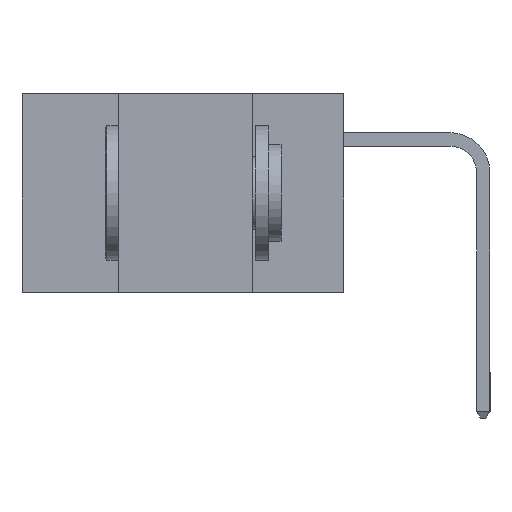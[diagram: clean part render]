
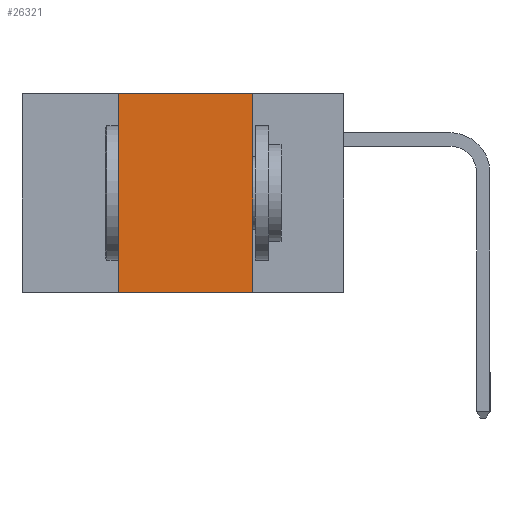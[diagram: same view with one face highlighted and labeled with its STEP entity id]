
A CAD part, left-side view. The second image highlights one B-rep face of the part: STEP entity #26321.
In plain terms, the highlighted planar face has unit normal (-1, 0, 0).
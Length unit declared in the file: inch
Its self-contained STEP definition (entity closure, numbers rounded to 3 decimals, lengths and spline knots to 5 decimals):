
#24 = LINE ( 'NONE', #15750, #25617 ) ;
#314 = FACE_OUTER_BOUND ( 'NONE', #26696, .T. ) ;
#1170 = EDGE_CURVE ( 'NONE', #27812, #8959, #24, .T. ) ;
#1636 = ORIENTED_EDGE ( 'NONE', *, *, #12456, .F. ) ;
#3092 = EDGE_CURVE ( 'NONE', #28679, #8959, #13133, .T. ) ;
#3918 = ORIENTED_EDGE ( 'NONE', *, *, #3092, .T. ) ;
#4288 = DIRECTION ( 'NONE',  ( 0., 0., -1. ) ) ;
#5639 = VECTOR ( 'NONE', #26597, 39.37008 ) ;
#6387 = LINE ( 'NONE', #10277, #5639 ) ;
#6411 = DIRECTION ( 'NONE',  ( 0., 0., 1. ) ) ;
#7073 = CARTESIAN_POINT ( 'NONE',  ( 0., 0.6, 0. ) ) ;
#8651 = CARTESIAN_POINT ( 'NONE',  ( 0., 0.42, 0. ) ) ;
#8959 = VERTEX_POINT ( 'NONE', #29055 ) ;
#10277 = CARTESIAN_POINT ( 'NONE',  ( 0., 0.6, 0. ) ) ;
#11263 = VECTOR ( 'NONE', #6411, 39.37008 ) ;
#11785 = DIRECTION ( 'NONE',  ( 1., 0., 0. ) ) ;
#12456 = EDGE_CURVE ( 'NONE', #28679, #15115, #17439, .T. ) ;
#12586 = DIRECTION ( 'NONE',  ( 0., -1., 0. ) ) ;
#13133 = LINE ( 'NONE', #24733, #24823 ) ;
#15115 = VERTEX_POINT ( 'NONE', #21785 ) ;
#15202 = EDGE_CURVE ( 'NONE', #15115, #27812, #6387, .T. ) ;
#15750 = CARTESIAN_POINT ( 'NONE',  ( 0., 0.17, 0. ) ) ;
#16474 = DIRECTION ( 'NONE',  ( 0., 0., -1. ) ) ;
#17439 = LINE ( 'NONE', #8651, #11263 ) ;
#21056 = PLANE ( 'NONE',  #28316 ) ;
#21134 = CARTESIAN_POINT ( 'NONE',  ( 0., 0.42, -0.37 ) ) ;
#21785 = CARTESIAN_POINT ( 'NONE',  ( 0., 0.42, 0. ) ) ;
#22407 = CARTESIAN_POINT ( 'NONE',  ( 0., 0.17, 0. ) ) ;
#24733 = CARTESIAN_POINT ( 'NONE',  ( 0., 0.6, -0.37 ) ) ;
#24823 = VECTOR ( 'NONE', #12586, 39.37008 ) ;
#25617 = VECTOR ( 'NONE', #4288, 39.37008 ) ;
#26321 = ADVANCED_FACE ( 'NONE', ( #314 ), #21056, .F. ) ;
#26597 = DIRECTION ( 'NONE',  ( 0., -1., 0. ) ) ;
#26696 = EDGE_LOOP ( 'NONE', ( #29336, #28845, #1636, #3918 ) ) ;
#27812 = VERTEX_POINT ( 'NONE', #22407 ) ;
#28316 = AXIS2_PLACEMENT_3D ( 'NONE', #7073, #11785, #16474 ) ;
#28679 = VERTEX_POINT ( 'NONE', #21134 ) ;
#28845 = ORIENTED_EDGE ( 'NONE', *, *, #15202, .F. ) ;
#29055 = CARTESIAN_POINT ( 'NONE',  ( 0., 0.17, -0.37 ) ) ;
#29336 = ORIENTED_EDGE ( 'NONE', *, *, #1170, .F. ) ;
